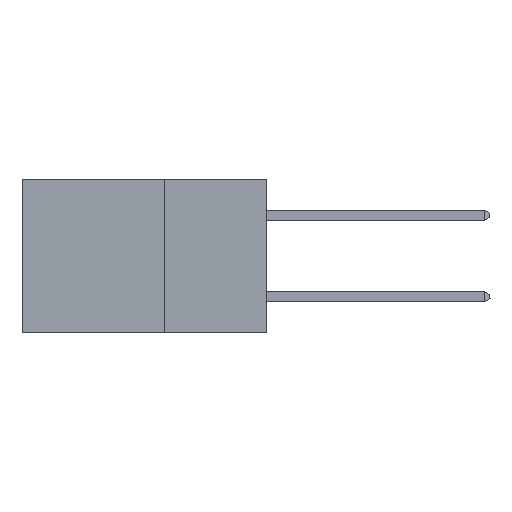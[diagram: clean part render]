
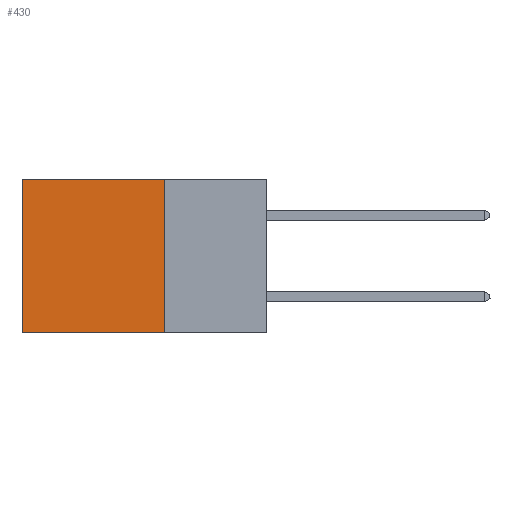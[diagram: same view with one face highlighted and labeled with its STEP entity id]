
A CAD part, left-side view. The second image highlights one B-rep face of the part: STEP entity #430.
In plain terms, the highlighted planar face has unit normal (-1, 0, 0).
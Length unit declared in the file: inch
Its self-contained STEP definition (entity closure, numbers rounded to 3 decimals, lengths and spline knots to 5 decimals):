
#39 = VECTOR ( 'NONE', #15395, 39.37008 ) ;
#430 = ADVANCED_FACE ( 'NONE', ( #5029 ), #8143, .F. ) ;
#779 = CARTESIAN_POINT ( 'NONE',  ( 0.2875, 0.6, 0. ) ) ;
#982 = ORIENTED_EDGE ( 'NONE', *, *, #15222, .T. ) ;
#1584 = CARTESIAN_POINT ( 'NONE',  ( 0.2875, 0.25, -0.375 ) ) ;
#2469 = DIRECTION ( 'NONE',  ( 0., 1., 0. ) ) ;
#2608 = DIRECTION ( 'NONE',  ( 0., 0., -1. ) ) ;
#2738 = ORIENTED_EDGE ( 'NONE', *, *, #3678, .F. ) ;
#2927 = EDGE_CURVE ( 'NONE', #8203, #17685, #4497, .T. ) ;
#3678 = EDGE_CURVE ( 'NONE', #5889, #18339, #5635, .T. ) ;
#3880 = ORIENTED_EDGE ( 'NONE', *, *, #11732, .F. ) ;
#4497 = LINE ( 'NONE', #12873, #16766 ) ;
#5029 = FACE_OUTER_BOUND ( 'NONE', #10065, .T. ) ;
#5046 = CARTESIAN_POINT ( 'NONE',  ( 0.2875, 0.25, 0. ) ) ;
#5242 = CARTESIAN_POINT ( 'NONE',  ( 0.2875, 0.25, -0.375 ) ) ;
#5635 = LINE ( 'NONE', #1584, #15359 ) ;
#5889 = VERTEX_POINT ( 'NONE', #5046 ) ;
#6093 = VECTOR ( 'NONE', #2469, 39.37008 ) ;
#8143 = PLANE ( 'NONE',  #17419 ) ;
#8203 = VERTEX_POINT ( 'NONE', #779 ) ;
#9348 = CARTESIAN_POINT ( 'NONE',  ( 0.2875, 0.25, -0.375 ) ) ;
#9603 = DIRECTION ( 'NONE',  ( 1., 0., 0. ) ) ;
#9937 = LINE ( 'NONE', #11025, #6093 ) ;
#10065 = EDGE_LOOP ( 'NONE', ( #10433, #3880, #2738, #982 ) ) ;
#10433 = ORIENTED_EDGE ( 'NONE', *, *, #2927, .T. ) ;
#11025 = CARTESIAN_POINT ( 'NONE',  ( 0.2875, 0.25, 0. ) ) ;
#11732 = EDGE_CURVE ( 'NONE', #18339, #17685, #17084, .T. ) ;
#12140 = CARTESIAN_POINT ( 'NONE',  ( 0.2875, 0.25, -0.375 ) ) ;
#12338 = CARTESIAN_POINT ( 'NONE',  ( 0.2875, 0.6, -0.375 ) ) ;
#12873 = CARTESIAN_POINT ( 'NONE',  ( 0.2875, 0.6, -0.375 ) ) ;
#13038 = DIRECTION ( 'NONE',  ( 0., 0., -1. ) ) ;
#15222 = EDGE_CURVE ( 'NONE', #5889, #8203, #9937, .T. ) ;
#15263 = DIRECTION ( 'NONE',  ( 0., 0., -1. ) ) ;
#15359 = VECTOR ( 'NONE', #13038, 39.37008 ) ;
#15395 = DIRECTION ( 'NONE',  ( 0., 1., 0. ) ) ;
#16766 = VECTOR ( 'NONE', #2608, 39.37008 ) ;
#17084 = LINE ( 'NONE', #12140, #39 ) ;
#17419 = AXIS2_PLACEMENT_3D ( 'NONE', #5242, #9603, #15263 ) ;
#17685 = VERTEX_POINT ( 'NONE', #12338 ) ;
#18339 = VERTEX_POINT ( 'NONE', #9348 ) ;
